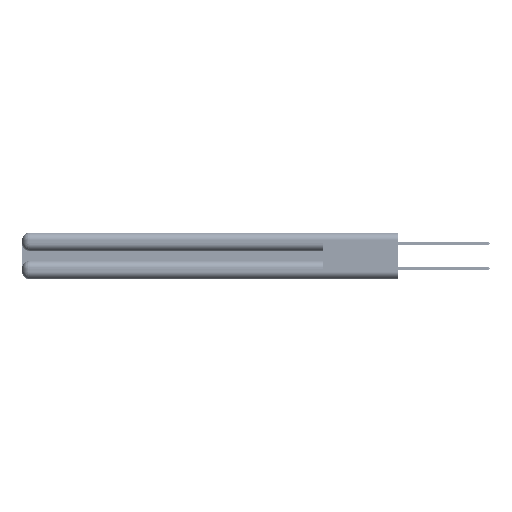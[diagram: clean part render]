
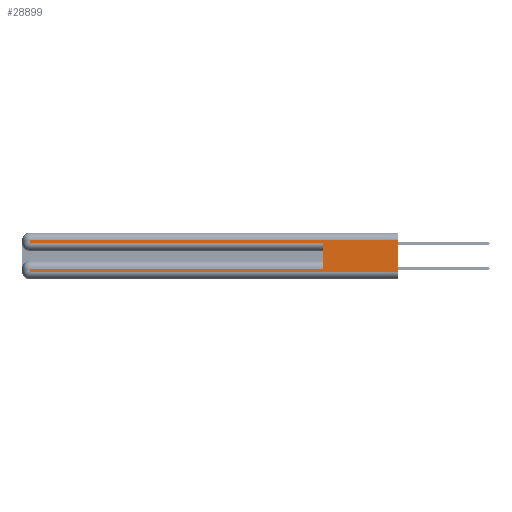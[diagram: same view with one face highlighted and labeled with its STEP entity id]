
A CAD part, left-side view. The second image highlights one B-rep face of the part: STEP entity #28899.
In plain terms, the highlighted planar face has unit normal (-1, 0, 0).
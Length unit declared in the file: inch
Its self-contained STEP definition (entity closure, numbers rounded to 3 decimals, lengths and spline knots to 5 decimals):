
#1279 = CARTESIAN_POINT ( 'NONE',  ( 0., 2.94, 0.285 ) ) ;
#1913 = EDGE_CURVE ( 'NONE', #18250, #42569, #56290, .T. ) ;
#2505 = DIRECTION ( 'NONE',  ( 1., 0., 0. ) ) ;
#4373 = CARTESIAN_POINT ( 'NONE',  ( 0., 0., 0.31 ) ) ;
#4724 = CARTESIAN_POINT ( 'NONE',  ( 0., 2.94, 0.085 ) ) ;
#5060 = CARTESIAN_POINT ( 'NONE',  ( 0., 0., 0.37 ) ) ;
#5073 = VERTEX_POINT ( 'NONE', #4724 ) ;
#5307 = ORIENTED_EDGE ( 'NONE', *, *, #45861, .T. ) ;
#5866 = LINE ( 'NONE', #17944, #27923 ) ;
#6327 = CARTESIAN_POINT ( 'NONE',  ( 0., 2.94, 0.37 ) ) ;
#6816 = VERTEX_POINT ( 'NONE', #1279 ) ;
#8709 = AXIS2_PLACEMENT_3D ( 'NONE', #46290, #2505, #33373 ) ;
#9211 = EDGE_CURVE ( 'NONE', #6816, #42569, #5866, .T. ) ;
#11269 = EDGE_CURVE ( 'NONE', #22455, #48732, #35755, .T. ) ;
#12958 = FACE_OUTER_BOUND ( 'NONE', #48425, .T. ) ;
#13955 = CARTESIAN_POINT ( 'NONE',  ( 0., 2.94, 0.37 ) ) ;
#14428 = VECTOR ( 'NONE', #45839, 39.37008 ) ;
#14595 = CARTESIAN_POINT ( 'NONE',  ( 0., 0.6, 0.145 ) ) ;
#15811 = ORIENTED_EDGE ( 'NONE', *, *, #41400, .F. ) ;
#15838 = LINE ( 'NONE', #5060, #26202 ) ;
#17944 = CARTESIAN_POINT ( 'NONE',  ( 0., 0., 0.285 ) ) ;
#18250 = VERTEX_POINT ( 'NONE', #32959 ) ;
#18403 = DIRECTION ( 'NONE',  ( 0., 0., -1. ) ) ;
#18617 = CARTESIAN_POINT ( 'NONE',  ( 0., 0., 0.085 ) ) ;
#18999 = ORIENTED_EDGE ( 'NONE', *, *, #36024, .T. ) ;
#20187 = LINE ( 'NONE', #13955, #42122 ) ;
#20756 = CARTESIAN_POINT ( 'NONE',  ( 0., 0., 0.06 ) ) ;
#21192 = CARTESIAN_POINT ( 'NONE',  ( 0., 0., 0.31 ) ) ;
#21443 = VECTOR ( 'NONE', #54054, 39.37008 ) ;
#21787 = EDGE_CURVE ( 'NONE', #5073, #22455, #26158, .T. ) ;
#22455 = VERTEX_POINT ( 'NONE', #28997 ) ;
#23008 = CARTESIAN_POINT ( 'NONE',  ( 0., 2.94, 0.31 ) ) ;
#26158 = LINE ( 'NONE', #6327, #14428 ) ;
#26202 = VECTOR ( 'NONE', #31488, 39.37008 ) ;
#27512 = CARTESIAN_POINT ( 'NONE',  ( 0., 0.6, 0.285 ) ) ;
#27923 = VECTOR ( 'NONE', #31084, 39.37008 ) ;
#28899 = ADVANCED_FACE ( 'NONE', ( #12958 ), #55075, .F. ) ;
#28997 = CARTESIAN_POINT ( 'NONE',  ( 0., 2.94, 0.06 ) ) ;
#31084 = DIRECTION ( 'NONE',  ( 0., -1., 0. ) ) ;
#31488 = DIRECTION ( 'NONE',  ( 0., 0., -1. ) ) ;
#31848 = VERTEX_POINT ( 'NONE', #21192 ) ;
#32931 = LINE ( 'NONE', #4373, #54719 ) ;
#32959 = CARTESIAN_POINT ( 'NONE',  ( 0., 0.6, 0.085 ) ) ;
#33373 = DIRECTION ( 'NONE',  ( 0., 0., -1. ) ) ;
#35755 = LINE ( 'NONE', #44586, #47314 ) ;
#36024 = EDGE_CURVE ( 'NONE', #18250, #5073, #56309, .T. ) ;
#36504 = DIRECTION ( 'NONE',  ( 0., 1., 0. ) ) ;
#38047 = DIRECTION ( 'NONE',  ( 0., 1., 0. ) ) ;
#40080 = ORIENTED_EDGE ( 'NONE', *, *, #11269, .T. ) ;
#41400 = EDGE_CURVE ( 'NONE', #31848, #48732, #15838, .T. ) ;
#41496 = VERTEX_POINT ( 'NONE', #23008 ) ;
#42122 = VECTOR ( 'NONE', #18403, 39.37008 ) ;
#42569 = VERTEX_POINT ( 'NONE', #27512 ) ;
#44586 = CARTESIAN_POINT ( 'NONE',  ( 0., 0., 0.06 ) ) ;
#45707 = ORIENTED_EDGE ( 'NONE', *, *, #21787, .T. ) ;
#45839 = DIRECTION ( 'NONE',  ( 0., 0., -1. ) ) ;
#45861 = EDGE_CURVE ( 'NONE', #31848, #41496, #32931, .T. ) ;
#46290 = CARTESIAN_POINT ( 'NONE',  ( 0., 0., 0.37 ) ) ;
#46776 = ORIENTED_EDGE ( 'NONE', *, *, #50359, .T. ) ;
#47314 = VECTOR ( 'NONE', #48988, 39.37008 ) ;
#48425 = EDGE_LOOP ( 'NONE', ( #15811, #5307, #46776, #54834, #52595, #18999, #45707, #40080 ) ) ;
#48732 = VERTEX_POINT ( 'NONE', #20756 ) ;
#48988 = DIRECTION ( 'NONE',  ( 0., -1., 0. ) ) ;
#50359 = EDGE_CURVE ( 'NONE', #41496, #6816, #20187, .T. ) ;
#52595 = ORIENTED_EDGE ( 'NONE', *, *, #1913, .F. ) ;
#54054 = DIRECTION ( 'NONE',  ( 0., 0., 1. ) ) ;
#54719 = VECTOR ( 'NONE', #38047, 39.37008 ) ;
#54834 = ORIENTED_EDGE ( 'NONE', *, *, #9211, .T. ) ;
#54967 = VECTOR ( 'NONE', #36504, 39.37008 ) ;
#55075 = PLANE ( 'NONE',  #8709 ) ;
#56290 = LINE ( 'NONE', #14595, #21443 ) ;
#56309 = LINE ( 'NONE', #18617, #54967 ) ;
